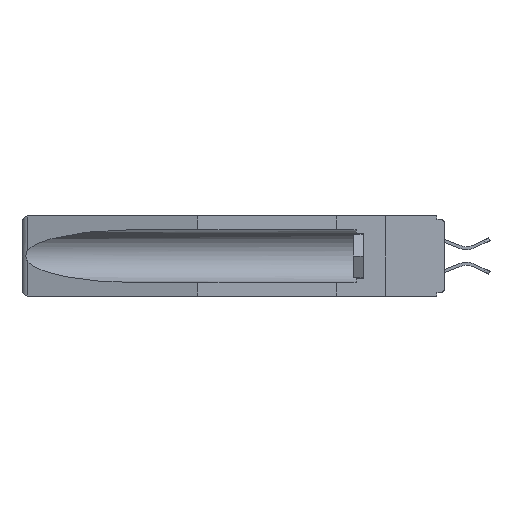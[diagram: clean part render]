
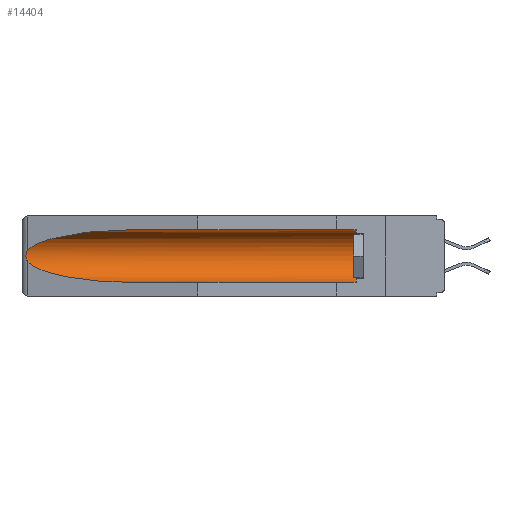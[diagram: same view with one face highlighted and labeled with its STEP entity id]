
A CAD part, left-side view. The second image highlights one B-rep face of the part: STEP entity #14404.
In plain terms, the highlighted cylindrical face has radius 2.857 mm (diameter 5.715 mm), a partial arc.
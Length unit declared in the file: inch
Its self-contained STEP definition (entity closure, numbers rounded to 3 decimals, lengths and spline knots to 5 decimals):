
#800 = VERTEX_POINT ( 'NONE', #3907 ) ;
#1005 = CARTESIAN_POINT ( 'NONE',  ( 0.25451, 1.48313, -0.24835 ) ) ;
#1173 = CARTESIAN_POINT ( 'NONE',  ( 0.2673, 1.53269, -0.17917 ) ) ;
#1186 = VERTEX_POINT ( 'NONE', #19192 ) ;
#1534 = CARTESIAN_POINT ( 'NONE',  ( 0.155, 1.07973, -0.284 ) ) ;
#2267 = DIRECTION ( 'NONE',  ( 0., 1., 0. ) ) ;
#2730 = CARTESIAN_POINT ( 'NONE',  ( 0.26597, 1.5296, -0.19026 ) ) ;
#2962 =( BOUNDED_CURVE ( )  B_SPLINE_CURVE ( 3, ( #20358, #1005, #5714, #18845 ),
 .UNSPECIFIED., .F., .F. ) 
 B_SPLINE_CURVE_WITH_KNOTS ( ( 4, 4 ),
 ( 0.1948, 1.5708 ),
 .UNSPECIFIED. ) 
 CURVE ( )  GEOMETRIC_REPRESENTATION_ITEM ( )  RATIONAL_B_SPLINE_CURVE ( ( 1., 0.848, 0.848, 1. ) ) 
 REPRESENTATION_ITEM ( '' )  );
#3511 = FACE_OUTER_BOUND ( 'NONE', #3526, .T. ) ;
#3526 = EDGE_LOOP ( 'NONE', ( #12746, #7228, #10634, #18578, #11558, #8795 ) ) ;
#3611 = B_SPLINE_CURVE_WITH_KNOTS ( 'NONE', 3,
 ( #4253, #14076, #20744, #19222, #7573, #9331, #1173, #9405, #2730, #20883 ),
 .UNSPECIFIED., .F., .F.,
 ( 4, 2, 2, 2, 4 ),
 ( 0., 0.00029, 0.00058, 0.00087, 0.00117 ),
 .UNSPECIFIED. ) ;
#3646 = VECTOR ( 'NONE', #13834, 39.37008 ) ;
#3907 = CARTESIAN_POINT ( 'NONE',  ( 0.26537, 1.52718, -0.19328 ) ) ;
#4253 = CARTESIAN_POINT ( 'NONE',  ( 0.26537, 1.52718, -0.14972 ) ) ;
#5376 = CIRCLE ( 'NONE', #14187, 0.1125 ) ;
#5714 = CARTESIAN_POINT ( 'NONE',  ( 0.21114, 1.30732, -0.284 ) ) ;
#5732 = LINE ( 'NONE', #7235, #3646 ) ;
#6700 = CARTESIAN_POINT ( 'NONE',  ( 0.155, -0.30754, -0.1715 ) ) ;
#7093 = CARTESIAN_POINT ( 'NONE',  ( 0.21114, 1.30732, -0.059 ) ) ;
#7170 = CARTESIAN_POINT ( 'NONE',  ( 0.155, 1.07973, -0.059 ) ) ;
#7228 = ORIENTED_EDGE ( 'NONE', *, *, #16286, .T. ) ;
#7235 = CARTESIAN_POINT ( 'NONE',  ( 0.155, -0.30754, -0.059 ) ) ;
#7573 = CARTESIAN_POINT ( 'NONE',  ( 0.2675, 1.53308, -0.16763 ) ) ;
#8168 = EDGE_CURVE ( 'NONE', #10749, #19057, #5732, .T. ) ;
#8795 = ORIENTED_EDGE ( 'NONE', *, *, #8168, .T. ) ;
#9270 = DIRECTION ( 'NONE',  ( 0., -1., 0. ) ) ;
#9331 = CARTESIAN_POINT ( 'NONE',  ( 0.2675, 1.53308, -0.17534 ) ) ;
#9405 = CARTESIAN_POINT ( 'NONE',  ( 0.26655, 1.53094, -0.18657 ) ) ;
#10277 = VERTEX_POINT ( 'NONE', #15361 ) ;
#10634 = ORIENTED_EDGE ( 'NONE', *, *, #13356, .T. ) ;
#10749 = VERTEX_POINT ( 'NONE', #17485 ) ;
#11558 = ORIENTED_EDGE ( 'NONE', *, *, #19480, .T. ) ;
#12087 = CARTESIAN_POINT ( 'NONE',  ( 0.155, -0.30754, -0.284 ) ) ;
#12746 = ORIENTED_EDGE ( 'NONE', *, *, #15818, .T. ) ;
#12835 = CARTESIAN_POINT ( 'NONE',  ( 0.155, 0.126, -0.1715 ) ) ;
#13283 = CYLINDRICAL_SURFACE ( 'NONE', #14921, 0.1125 ) ;
#13356 = EDGE_CURVE ( 'NONE', #800, #20133, #2962, .T. ) ;
#13834 = DIRECTION ( 'NONE',  ( 0., 1., 0. ) ) ;
#13859 = LINE ( 'NONE', #12087, #19243 ) ;
#14076 = CARTESIAN_POINT ( 'NONE',  ( 0.26597, 1.52961, -0.15275 ) ) ;
#14187 = AXIS2_PLACEMENT_3D ( 'NONE', #12835, #9270, #20752 ) ;
#14404 = ADVANCED_FACE ( 'NONE', ( #3511 ), #13283, .F. ) ;
#14896 = DIRECTION ( 'NONE',  ( 0., 1., 0. ) ) ;
#14921 = AXIS2_PLACEMENT_3D ( 'NONE', #6700, #14896, #16613 ) ;
#15361 = CARTESIAN_POINT ( 'NONE',  ( 0.155, 0.126, -0.284 ) ) ;
#15818 = EDGE_CURVE ( 'NONE', #19057, #1186, #17596, .T. ) ;
#16286 = EDGE_CURVE ( 'NONE', #1186, #800, #3611, .T. ) ;
#16613 = DIRECTION ( 'NONE',  ( 0., 0., 1. ) ) ;
#16856 = CARTESIAN_POINT ( 'NONE',  ( 0.25451, 1.48313, -0.09465 ) ) ;
#17086 = CARTESIAN_POINT ( 'NONE',  ( 0.26537, 1.52718, -0.14972 ) ) ;
#17485 = CARTESIAN_POINT ( 'NONE',  ( 0.155, 0.126, -0.059 ) ) ;
#17596 =( BOUNDED_CURVE ( )  B_SPLINE_CURVE ( 3, ( #7170, #7093, #16856, #17086 ),
 .UNSPECIFIED., .F., .F. ) 
 B_SPLINE_CURVE_WITH_KNOTS ( ( 4, 4 ),
 ( 4.71239, 6.08839 ),
 .UNSPECIFIED. ) 
 CURVE ( )  GEOMETRIC_REPRESENTATION_ITEM ( )  RATIONAL_B_SPLINE_CURVE ( ( 1., 0.848, 0.848, 1. ) ) 
 REPRESENTATION_ITEM ( '' )  );
#18255 = CARTESIAN_POINT ( 'NONE',  ( 0.155, 1.07973, -0.059 ) ) ;
#18578 = ORIENTED_EDGE ( 'NONE', *, *, #19208, .F. ) ;
#18845 = CARTESIAN_POINT ( 'NONE',  ( 0.155, 1.07973, -0.284 ) ) ;
#19057 = VERTEX_POINT ( 'NONE', #18255 ) ;
#19192 = CARTESIAN_POINT ( 'NONE',  ( 0.26537, 1.52718, -0.14972 ) ) ;
#19208 = EDGE_CURVE ( 'NONE', #10277, #20133, #13859, .T. ) ;
#19222 = CARTESIAN_POINT ( 'NONE',  ( 0.2673, 1.5327, -0.16383 ) ) ;
#19243 = VECTOR ( 'NONE', #2267, 39.37008 ) ;
#19480 = EDGE_CURVE ( 'NONE', #10277, #10749, #5376, .T. ) ;
#20133 = VERTEX_POINT ( 'NONE', #1534 ) ;
#20358 = CARTESIAN_POINT ( 'NONE',  ( 0.26537, 1.52718, -0.19328 ) ) ;
#20744 = CARTESIAN_POINT ( 'NONE',  ( 0.26654, 1.53092, -0.15636 ) ) ;
#20752 = DIRECTION ( 'NONE',  ( 0., 0., 1. ) ) ;
#20883 = CARTESIAN_POINT ( 'NONE',  ( 0.26537, 1.52718, -0.19328 ) ) ;
